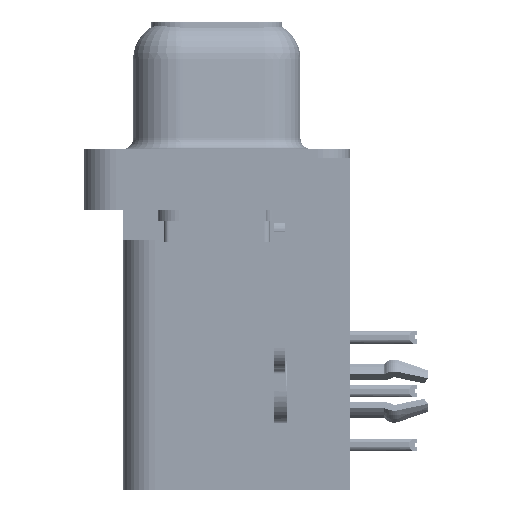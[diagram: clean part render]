
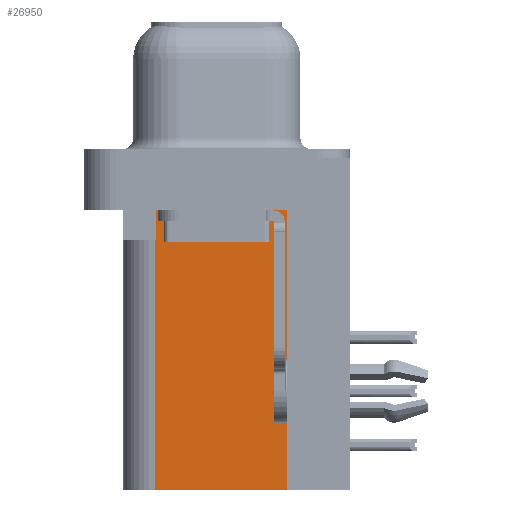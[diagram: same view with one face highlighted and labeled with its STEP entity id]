
A CAD part, left-side view. The second image highlights one B-rep face of the part: STEP entity #26950.
In plain terms, the highlighted planar face has unit normal (-1, 0, 0).
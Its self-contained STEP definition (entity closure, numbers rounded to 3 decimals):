
#4204 = ORIENTED_EDGE ( 'NONE', *, *, #25939, .F. ) ;
#4736 = FACE_OUTER_BOUND ( 'NONE', #35127, .T. ) ;
#6521 = CARTESIAN_POINT ( 'NONE',  ( 3.79, -3.295, -15.7 ) ) ;
#6707 = VERTEX_POINT ( 'NONE', #48437 ) ;
#9211 = VECTOR ( 'NONE', #18456, 1000. ) ;
#9706 = ORIENTED_EDGE ( 'NONE', *, *, #31675, .T. ) ;
#10583 = CARTESIAN_POINT ( 'NONE',  ( 3.79, 2.925, -3.9 ) ) ;
#10602 = DIRECTION ( 'NONE',  ( 0., 0., -1. ) ) ;
#11476 = VERTEX_POINT ( 'NONE', #29325 ) ;
#14893 = VECTOR ( 'NONE', #28993, 1000. ) ;
#15322 = CARTESIAN_POINT ( 'NONE',  ( 3.79, 2.895, -3.9 ) ) ;
#15534 = VERTEX_POINT ( 'NONE', #10583 ) ;
#16403 = CARTESIAN_POINT ( 'NONE',  ( 3.79, 2.925, -15.7 ) ) ;
#16639 = EDGE_CURVE ( 'NONE', #41338, #15534, #52811, .T. ) ;
#18456 = DIRECTION ( 'NONE',  ( 0., 0., 1. ) ) ;
#22284 = ORIENTED_EDGE ( 'NONE', *, *, #24144, .T. ) ;
#22384 = LINE ( 'NONE', #44644, #33792 ) ;
#22551 = CARTESIAN_POINT ( 'NONE',  ( 3.79, -3.295, -15.7 ) ) ;
#22888 = CARTESIAN_POINT ( 'NONE',  ( 3.79, 0., -3.9 ) ) ;
#23533 = DIRECTION ( 'NONE',  ( 0., 0., -1. ) ) ;
#24144 = EDGE_CURVE ( 'NONE', #43010, #36274, #52815, .T. ) ;
#24853 = CARTESIAN_POINT ( 'NONE',  ( 3.79, -3.295, -2.5 ) ) ;
#25939 = EDGE_CURVE ( 'NONE', #43010, #6707, #27496, .T. ) ;
#26223 = LINE ( 'NONE', #16403, #37578 ) ;
#26950 = ADVANCED_FACE ( 'NONE', ( #4736 ), #27521, .F. ) ;
#27496 = LINE ( 'NONE', #48457, #37515 ) ;
#27521 = PLANE ( 'NONE',  #30236 ) ;
#28129 = ORIENTED_EDGE ( 'NONE', *, *, #36866, .F. ) ;
#28993 = DIRECTION ( 'NONE',  ( 0., 1., 0. ) ) ;
#29325 = CARTESIAN_POINT ( 'NONE',  ( 3.79, 2.895, -2.5 ) ) ;
#30236 = AXIS2_PLACEMENT_3D ( 'NONE', #31867, #36131, #10602 ) ;
#31675 = EDGE_CURVE ( 'NONE', #11476, #41338, #22384, .T. ) ;
#31867 = CARTESIAN_POINT ( 'NONE',  ( 3.79, -3.295, -15.7 ) ) ;
#33792 = VECTOR ( 'NONE', #23533, 1000. ) ;
#34122 = ORIENTED_EDGE ( 'NONE', *, *, #16639, .T. ) ;
#35127 = EDGE_LOOP ( 'NONE', ( #46329, #9706, #34122, #28129, #4204, #22284 ) ) ;
#36131 = DIRECTION ( 'NONE',  ( 1., 0., 0. ) ) ;
#36274 = VERTEX_POINT ( 'NONE', #52456 ) ;
#36866 = EDGE_CURVE ( 'NONE', #6707, #15534, #26223, .T. ) ;
#37498 = EDGE_CURVE ( 'NONE', #36274, #11476, #48620, .T. ) ;
#37515 = VECTOR ( 'NONE', #48641, 1000. ) ;
#37578 = VECTOR ( 'NONE', #49822, 1000. ) ;
#41338 = VERTEX_POINT ( 'NONE', #15322 ) ;
#41721 = VECTOR ( 'NONE', #48221, 1000. ) ;
#43010 = VERTEX_POINT ( 'NONE', #6521 ) ;
#44644 = CARTESIAN_POINT ( 'NONE',  ( 3.79, 2.895, -3.9 ) ) ;
#46329 = ORIENTED_EDGE ( 'NONE', *, *, #37498, .T. ) ;
#48221 = DIRECTION ( 'NONE',  ( 0., 1., 0. ) ) ;
#48437 = CARTESIAN_POINT ( 'NONE',  ( 3.79, 2.925, -15.7 ) ) ;
#48457 = CARTESIAN_POINT ( 'NONE',  ( 3.79, -3.295, -15.7 ) ) ;
#48620 = LINE ( 'NONE', #24853, #14893 ) ;
#48641 = DIRECTION ( 'NONE',  ( 0., 1., 0. ) ) ;
#49822 = DIRECTION ( 'NONE',  ( 0., 0., 1. ) ) ;
#52456 = CARTESIAN_POINT ( 'NONE',  ( 3.79, -3.295, -2.5 ) ) ;
#52811 = LINE ( 'NONE', #22888, #41721 ) ;
#52815 = LINE ( 'NONE', #22551, #9211 ) ;
